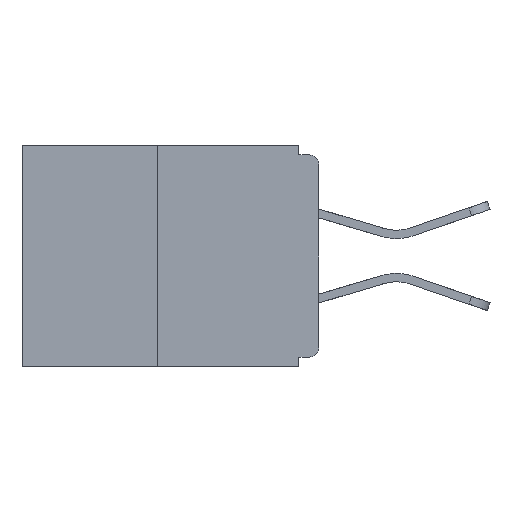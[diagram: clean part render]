
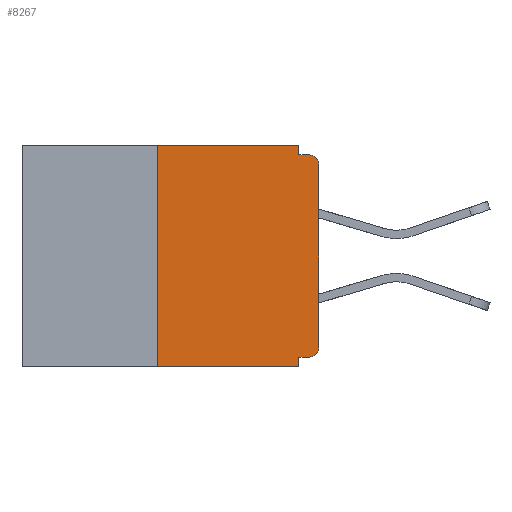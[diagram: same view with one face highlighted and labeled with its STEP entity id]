
A CAD part, left-side view. The second image highlights one B-rep face of the part: STEP entity #8267.
In plain terms, the highlighted planar face has unit normal (-1, 0, 0).
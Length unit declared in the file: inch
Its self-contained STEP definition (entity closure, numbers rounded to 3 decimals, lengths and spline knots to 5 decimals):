
#82 = VERTEX_POINT ( 'NONE', #374 ) ;
#134 = CIRCLE ( 'NONE', #5752, 0.015 ) ;
#249 = VERTEX_POINT ( 'NONE', #10088 ) ;
#281 = DIRECTION ( 'NONE',  ( 0., 0., -1. ) ) ;
#355 = CARTESIAN_POINT ( 'NONE',  ( 0., 0., -0.015 ) ) ;
#374 = CARTESIAN_POINT ( 'NONE',  ( 0., 0.25, -0.343 ) ) ;
#390 = AXIS2_PLACEMENT_3D ( 'NONE', #12216, #3026, #15172 ) ;
#605 = CARTESIAN_POINT ( 'NONE',  ( 0., 0.031, -0.328 ) ) ;
#1186 = CARTESIAN_POINT ( 'NONE',  ( 0., 0.46, -0.343 ) ) ;
#1489 = CARTESIAN_POINT ( 'NONE',  ( 0., 0.015, -0.015 ) ) ;
#1579 = CARTESIAN_POINT ( 'NONE',  ( 0., 0.031, -0.343 ) ) ;
#1908 = CARTESIAN_POINT ( 'NONE',  ( 0., 0.031, -0.343 ) ) ;
#1948 = LINE ( 'NONE', #4567, #4905 ) ;
#2261 = FACE_OUTER_BOUND ( 'NONE', #13061, .T. ) ;
#2361 = DIRECTION ( 'NONE',  ( 0., 0., -1. ) ) ;
#2519 = VERTEX_POINT ( 'NONE', #1579 ) ;
#2695 = VECTOR ( 'NONE', #10082, 39.37008 ) ;
#2880 = EDGE_CURVE ( 'NONE', #7719, #249, #11554, .T. ) ;
#2950 = CARTESIAN_POINT ( 'NONE',  ( 0., 0.015, -0.03 ) ) ;
#3026 = DIRECTION ( 'NONE',  ( 1., 0., 0. ) ) ;
#3553 = CARTESIAN_POINT ( 'NONE',  ( 0., 0.015, -0.313 ) ) ;
#3577 = ORIENTED_EDGE ( 'NONE', *, *, #2880, .T. ) ;
#3921 = CARTESIAN_POINT ( 'NONE',  ( 0., 0.25, 0. ) ) ;
#4190 = CARTESIAN_POINT ( 'NONE',  ( 0., 0.031, 0. ) ) ;
#4197 = ORIENTED_EDGE ( 'NONE', *, *, #8362, .T. ) ;
#4402 = LINE ( 'NONE', #12948, #4588 ) ;
#4503 = CARTESIAN_POINT ( 'NONE',  ( 0., 0., -0.03 ) ) ;
#4567 = CARTESIAN_POINT ( 'NONE',  ( 0., 0.46, 0. ) ) ;
#4588 = VECTOR ( 'NONE', #6880, 39.37008 ) ;
#4905 = VECTOR ( 'NONE', #5779, 39.37008 ) ;
#5148 = VERTEX_POINT ( 'NONE', #8875 ) ;
#5294 = LINE ( 'NONE', #3921, #2695 ) ;
#5437 = DIRECTION ( 'NONE',  ( 0., 0., -1. ) ) ;
#5752 = AXIS2_PLACEMENT_3D ( 'NONE', #2950, #11667, #5437 ) ;
#5779 = DIRECTION ( 'NONE',  ( 0., -1., 0. ) ) ;
#6058 = DIRECTION ( 'NONE',  ( 0., -1., 0. ) ) ;
#6157 = EDGE_CURVE ( 'NONE', #7719, #6181, #12823, .T. ) ;
#6181 = VERTEX_POINT ( 'NONE', #605 ) ;
#6671 = VECTOR ( 'NONE', #7804, 39.37008 ) ;
#6732 = EDGE_CURVE ( 'NONE', #8511, #5148, #1948, .T. ) ;
#6767 = VERTEX_POINT ( 'NONE', #4503 ) ;
#6880 = DIRECTION ( 'NONE',  ( 0., 0., 1. ) ) ;
#7137 = PLANE ( 'NONE',  #390 ) ;
#7166 = VECTOR ( 'NONE', #13730, 39.37008 ) ;
#7260 = LINE ( 'NONE', #1186, #11371 ) ;
#7707 = LINE ( 'NONE', #355, #8311 ) ;
#7719 = VERTEX_POINT ( 'NONE', #14113 ) ;
#7804 = DIRECTION ( 'NONE',  ( 0., 1., 0. ) ) ;
#7944 = ORIENTED_EDGE ( 'NONE', *, *, #11019, .T. ) ;
#7984 = EDGE_CURVE ( 'NONE', #5148, #13491, #15129, .T. ) ;
#8267 = ADVANCED_FACE ( 'NONE', ( #2261 ), #7137, .F. ) ;
#8311 = VECTOR ( 'NONE', #11298, 39.37008 ) ;
#8362 = EDGE_CURVE ( 'NONE', #6767, #13425, #134, .T. ) ;
#8440 = DIRECTION ( 'NONE',  ( -1., 0., 0. ) ) ;
#8511 = VERTEX_POINT ( 'NONE', #10775 ) ;
#8549 = VECTOR ( 'NONE', #281, 39.37008 ) ;
#8618 = ORIENTED_EDGE ( 'NONE', *, *, #14371, .F. ) ;
#8696 = EDGE_CURVE ( 'NONE', #82, #2519, #7260, .T. ) ;
#8875 = CARTESIAN_POINT ( 'NONE',  ( 0., 0.031, 0. ) ) ;
#9109 = CARTESIAN_POINT ( 'NONE',  ( 0., 0.031, -0.015 ) ) ;
#9706 = ORIENTED_EDGE ( 'NONE', *, *, #8696, .T. ) ;
#10082 = DIRECTION ( 'NONE',  ( 0., 0., 1. ) ) ;
#10088 = CARTESIAN_POINT ( 'NONE',  ( 0., 0., -0.313 ) ) ;
#10298 = LINE ( 'NONE', #1908, #7166 ) ;
#10555 = ORIENTED_EDGE ( 'NONE', *, *, #14814, .F. ) ;
#10775 = CARTESIAN_POINT ( 'NONE',  ( 0., 0.25, 0. ) ) ;
#11019 = EDGE_CURVE ( 'NONE', #249, #6767, #4402, .T. ) ;
#11298 = DIRECTION ( 'NONE',  ( 0., -1., 0. ) ) ;
#11371 = VECTOR ( 'NONE', #6058, 39.37008 ) ;
#11554 = CIRCLE ( 'NONE', #13339, 0.015 ) ;
#11667 = DIRECTION ( 'NONE',  ( -1., 0., 0. ) ) ;
#11868 = ORIENTED_EDGE ( 'NONE', *, *, #6732, .F. ) ;
#12216 = CARTESIAN_POINT ( 'NONE',  ( 0., 0.46, 0. ) ) ;
#12802 = EDGE_CURVE ( 'NONE', #6181, #2519, #10298, .T. ) ;
#12823 = LINE ( 'NONE', #14982, #6671 ) ;
#12948 = CARTESIAN_POINT ( 'NONE',  ( 0., 0., 0. ) ) ;
#13061 = EDGE_LOOP ( 'NONE', ( #11868, #10555, #9706, #13776, #13945, #3577, #7944, #4197, #8618, #13778 ) ) ;
#13339 = AXIS2_PLACEMENT_3D ( 'NONE', #3553, #8440, #2361 ) ;
#13425 = VERTEX_POINT ( 'NONE', #1489 ) ;
#13491 = VERTEX_POINT ( 'NONE', #9109 ) ;
#13730 = DIRECTION ( 'NONE',  ( 0., 0., -1. ) ) ;
#13776 = ORIENTED_EDGE ( 'NONE', *, *, #12802, .F. ) ;
#13778 = ORIENTED_EDGE ( 'NONE', *, *, #7984, .F. ) ;
#13945 = ORIENTED_EDGE ( 'NONE', *, *, #6157, .F. ) ;
#14113 = CARTESIAN_POINT ( 'NONE',  ( 0., 0.015, -0.328 ) ) ;
#14371 = EDGE_CURVE ( 'NONE', #13491, #13425, #7707, .T. ) ;
#14814 = EDGE_CURVE ( 'NONE', #82, #8511, #5294, .T. ) ;
#14982 = CARTESIAN_POINT ( 'NONE',  ( 0., 0., -0.328 ) ) ;
#15129 = LINE ( 'NONE', #4190, #8549 ) ;
#15172 = DIRECTION ( 'NONE',  ( 0., 0., -1. ) ) ;
